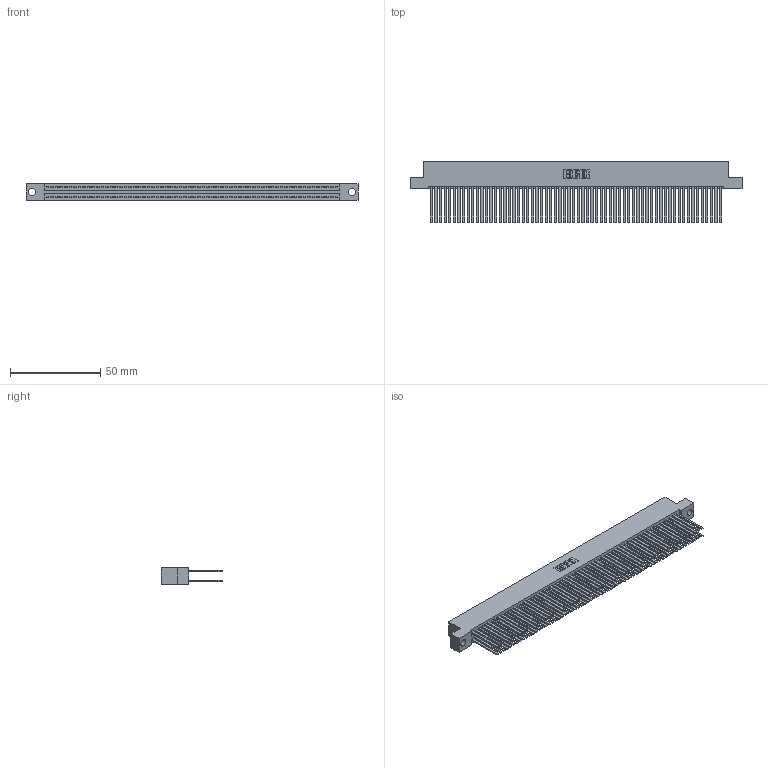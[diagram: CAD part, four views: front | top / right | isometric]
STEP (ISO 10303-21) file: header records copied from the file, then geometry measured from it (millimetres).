
FILE_DESCRIPTION (( 'STEP AP203' ), '1' );
FILE_NAME ('345-128-544-204.STEP', '2018-10-19T20:51:18', ( '' ), ( '' ), 'SwSTEP 2.0', 'SolidWorks 2016', '' );
FILE_SCHEMA (( 'CONFIG_CONTROL_DESIGN' ));
Length unit declared in the file: inch
Products named in the file (3): 345 Part_Flush Mounting Lugs - 0.156 Dia-TH; 345-128-544-204; 345-292-001_345-293-144
Assembly tree (129 placements, depth 2):
  345-128-544-204
    345 Part_Flush Mounting Lugs - 0.156 Dia-TH
    345-292-001_345-293-144  x128
Bounding box: 183.77 x 33.96 x 9.4 mm (x, y, z)
Volume: 19762.2 mm3; surface area: 34712.1 mm2
Topology: 129 solids, 129 shells, 5758 faces, 17109 edges, 11234 vertices
Faces by surface type: plane 3792, cylinder 1966
Entity records: 47073 total; most frequent: CARTESIAN_POINT 7868, ORIENTED_EDGE 7802, DIRECTION 6909, EDGE_CURVE 3901, LINE 3517, VECTOR 3517, VERTEX_POINT 2598, AXIS2_PLACEMENT_3D 1696
